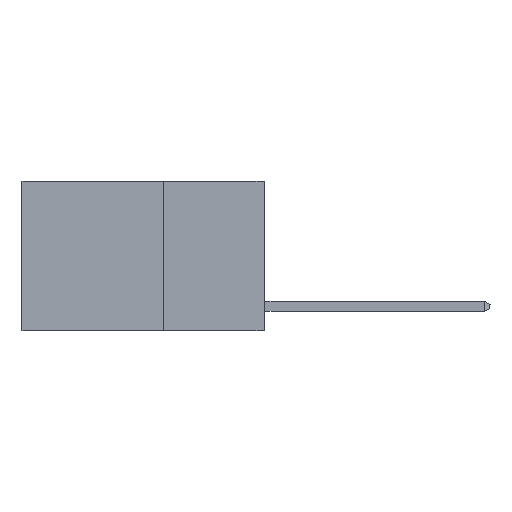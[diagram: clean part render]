
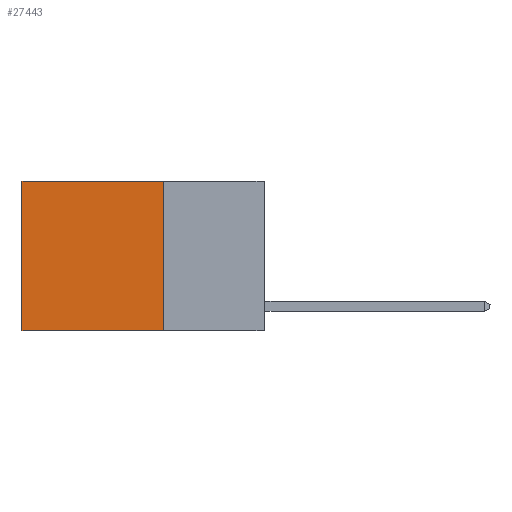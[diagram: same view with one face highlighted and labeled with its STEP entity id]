
A CAD part, left-side view. The second image highlights one B-rep face of the part: STEP entity #27443.
In plain terms, the highlighted planar face has unit normal (-1, 0, 0).
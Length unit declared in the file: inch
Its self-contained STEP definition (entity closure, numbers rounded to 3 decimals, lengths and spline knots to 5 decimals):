
#696 = DIRECTION ( 'NONE',  ( 0., 1., 0. ) ) ;
#1505 = EDGE_CURVE ( 'NONE', #23871, #11451, #12488, .T. ) ;
#1568 = DIRECTION ( 'NONE',  ( 0., 0., -1. ) ) ;
#1780 = DIRECTION ( 'NONE',  ( 0., 0., -1. ) ) ;
#1836 = ORIENTED_EDGE ( 'NONE', *, *, #25915, .T. ) ;
#2795 = ORIENTED_EDGE ( 'NONE', *, *, #22840, .F. ) ;
#2939 = DIRECTION ( 'NONE',  ( 0., 1., 0. ) ) ;
#3591 = VECTOR ( 'NONE', #23922, 39.37008 ) ;
#3764 = FACE_OUTER_BOUND ( 'NONE', #7042, .T. ) ;
#4078 = CARTESIAN_POINT ( 'NONE',  ( 0.2625, 0.6, 0. ) ) ;
#5346 = EDGE_CURVE ( 'NONE', #12041, #20443, #26692, .T. ) ;
#5566 = CARTESIAN_POINT ( 'NONE',  ( 0.2625, 0.25, -0.37 ) ) ;
#5676 = LINE ( 'NONE', #23524, #12464 ) ;
#7042 = EDGE_LOOP ( 'NONE', ( #20382, #2795, #13545, #1836 ) ) ;
#9698 = CARTESIAN_POINT ( 'NONE',  ( 0.2625, 0.25, -0.37 ) ) ;
#10474 = CARTESIAN_POINT ( 'NONE',  ( 0.2625, 0.6, -0.37 ) ) ;
#11451 = VERTEX_POINT ( 'NONE', #9698 ) ;
#12041 = VERTEX_POINT ( 'NONE', #4078 ) ;
#12464 = VECTOR ( 'NONE', #696, 39.37008 ) ;
#12488 = LINE ( 'NONE', #21419, #3591 ) ;
#12685 = PLANE ( 'NONE',  #24730 ) ;
#13545 = ORIENTED_EDGE ( 'NONE', *, *, #1505, .F. ) ;
#14466 = LINE ( 'NONE', #5566, #23646 ) ;
#17575 = CARTESIAN_POINT ( 'NONE',  ( 0.2625, 0.25, 0. ) ) ;
#20382 = ORIENTED_EDGE ( 'NONE', *, *, #5346, .T. ) ;
#20443 = VERTEX_POINT ( 'NONE', #10474 ) ;
#21419 = CARTESIAN_POINT ( 'NONE',  ( 0.2625, 0.25, 0. ) ) ;
#21615 = DIRECTION ( 'NONE',  ( 1., 0., 0. ) ) ;
#22840 = EDGE_CURVE ( 'NONE', #11451, #20443, #14466, .T. ) ;
#23524 = CARTESIAN_POINT ( 'NONE',  ( 0.2625, 0.25, 0. ) ) ;
#23646 = VECTOR ( 'NONE', #2939, 39.37008 ) ;
#23871 = VERTEX_POINT ( 'NONE', #17575 ) ;
#23922 = DIRECTION ( 'NONE',  ( 0., 0., -1. ) ) ;
#24050 = CARTESIAN_POINT ( 'NONE',  ( 0.2625, 0.6, 0. ) ) ;
#24259 = VECTOR ( 'NONE', #1780, 39.37008 ) ;
#24730 = AXIS2_PLACEMENT_3D ( 'NONE', #28368, #21615, #1568 ) ;
#25915 = EDGE_CURVE ( 'NONE', #23871, #12041, #5676, .T. ) ;
#26692 = LINE ( 'NONE', #24050, #24259 ) ;
#27443 = ADVANCED_FACE ( 'NONE', ( #3764 ), #12685, .F. ) ;
#28368 = CARTESIAN_POINT ( 'NONE',  ( 0.2625, 0.25, 0. ) ) ;
